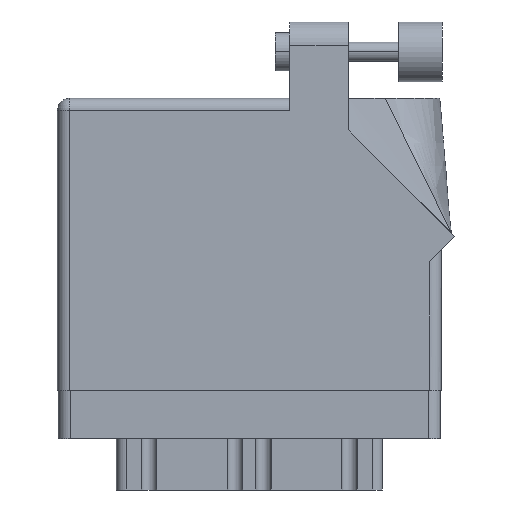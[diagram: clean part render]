
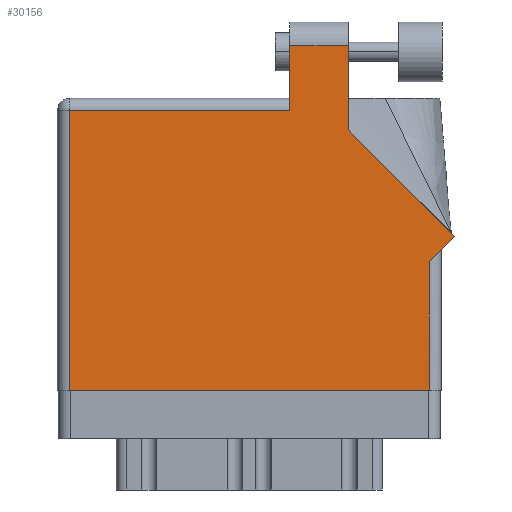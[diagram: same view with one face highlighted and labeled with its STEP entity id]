
A CAD part, front view. The second image highlights one B-rep face of the part: STEP entity #30156.
In plain terms, the highlighted face is planar.
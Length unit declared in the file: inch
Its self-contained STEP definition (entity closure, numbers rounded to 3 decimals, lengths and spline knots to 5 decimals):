
#331 = VECTOR ( 'NONE', #9564, 39.37008 ) ;
#849 = EDGE_CURVE ( 'NONE', #10601, #21095, #9066, .T. ) ;
#1721 = ORIENTED_EDGE ( 'NONE', *, *, #27608, .T. ) ;
#2180 = VECTOR ( 'NONE', #33624, 39.37008 ) ;
#2237 = ORIENTED_EDGE ( 'NONE', *, *, #849, .T. ) ;
#2464 = ORIENTED_EDGE ( 'NONE', *, *, #19576, .T. ) ;
#2592 = EDGE_CURVE ( 'NONE', #9937, #19014, #38317, .T. ) ;
#3768 = VECTOR ( 'NONE', #22594, 39.37008 ) ;
#4319 = CARTESIAN_POINT ( 'NONE',  ( 0.062, 0., 0. ) ) ;
#4365 = LINE ( 'NONE', #37009, #14744 ) ;
#4384 = CARTESIAN_POINT ( 'NONE',  ( 0., 1.53, 0. ) ) ;
#5187 = VERTEX_POINT ( 'NONE', #9441 ) ;
#5222 = ORIENTED_EDGE ( 'NONE', *, *, #8848, .T. ) ;
#5607 = CARTESIAN_POINT ( 'NONE',  ( 1.217, 1.53, 0. ) ) ;
#6119 = CARTESIAN_POINT ( 'NONE',  ( 0., 0., 0. ) ) ;
#6623 = EDGE_CURVE ( 'NONE', #9604, #5187, #30969, .T. ) ;
#6804 = CARTESIAN_POINT ( 'NONE',  ( 1.524, 1.36442, 0. ) ) ;
#7045 = LINE ( 'NONE', #19038, #22514 ) ;
#8455 = LINE ( 'NONE', #38750, #11746 ) ;
#8848 = EDGE_CURVE ( 'NONE', #19730, #20784, #20540, .T. ) ;
#9066 = LINE ( 'NONE', #6119, #2180 ) ;
#9441 = CARTESIAN_POINT ( 'NONE',  ( 1.524, 1.805, 0. ) ) ;
#9564 = DIRECTION ( 'NONE',  ( 0., 1., 0. ) ) ;
#9604 = VERTEX_POINT ( 'NONE', #27274 ) ;
#9704 = FACE_OUTER_BOUND ( 'NONE', #33405, .T. ) ;
#9937 = VERTEX_POINT ( 'NONE', #25664 ) ;
#10103 = CARTESIAN_POINT ( 'NONE',  ( 1.217, 1.468, 0. ) ) ;
#10601 = VERTEX_POINT ( 'NONE', #30463 ) ;
#10674 = VECTOR ( 'NONE', #21131, 39.37008 ) ;
#11167 = DIRECTION ( 'NONE',  ( 0.707, 0.707, 0. ) ) ;
#11746 = VECTOR ( 'NONE', #29871, 39.37008 ) ;
#12852 = DIRECTION ( 'NONE',  ( -1., 0., 0. ) ) ;
#13882 = EDGE_CURVE ( 'NONE', #20784, #26815, #8455, .T. ) ;
#14535 = ORIENTED_EDGE ( 'NONE', *, *, #6623, .T. ) ;
#14567 = DIRECTION ( 'NONE',  ( 0., 1., 0. ) ) ;
#14744 = VECTOR ( 'NONE', #22443, 39.37008 ) ;
#14761 = LINE ( 'NONE', #29287, #33579 ) ;
#15533 = AXIS2_PLACEMENT_3D ( 'NONE', #4384, #16373, #12852 ) ;
#16088 = DIRECTION ( 'NONE',  ( -0.707, 0.707, 0. ) ) ;
#16373 = DIRECTION ( 'NONE',  ( 0., 0., -1. ) ) ;
#19014 = VERTEX_POINT ( 'NONE', #31426 ) ;
#19038 = CARTESIAN_POINT ( 'NONE',  ( 2.08071, 0.80771, 0. ) ) ;
#19576 = EDGE_CURVE ( 'NONE', #26815, #10601, #28661, .T. ) ;
#19730 = VERTEX_POINT ( 'NONE', #38520 ) ;
#20540 = LINE ( 'NONE', #5607, #10674 ) ;
#20784 = VERTEX_POINT ( 'NONE', #10103 ) ;
#20887 = CARTESIAN_POINT ( 'NONE',  ( 1.948, 0., 0. ) ) ;
#21095 = VERTEX_POINT ( 'NONE', #20887 ) ;
#21131 = DIRECTION ( 'NONE',  ( 0., -1., 0. ) ) ;
#21914 = CARTESIAN_POINT ( 'NONE',  ( 0.062, 1.468, 0. ) ) ;
#22443 = DIRECTION ( 'NONE',  ( -1., 0., 0. ) ) ;
#22514 = VECTOR ( 'NONE', #16088, 39.37008 ) ;
#22594 = DIRECTION ( 'NONE',  ( 0., -1., 0. ) ) ;
#25664 = CARTESIAN_POINT ( 'NONE',  ( 1.948, 0.675, 0. ) ) ;
#26815 = VERTEX_POINT ( 'NONE', #21914 ) ;
#27274 = CARTESIAN_POINT ( 'NONE',  ( 1.524, 1.36442, 0. ) ) ;
#27559 = EDGE_CURVE ( 'NONE', #5187, #19730, #4365, .T. ) ;
#27608 = EDGE_CURVE ( 'NONE', #21095, #9937, #14761, .T. ) ;
#28661 = LINE ( 'NONE', #4319, #3768 ) ;
#28802 = ORIENTED_EDGE ( 'NONE', *, *, #13882, .T. ) ;
#29287 = CARTESIAN_POINT ( 'NONE',  ( 1.948, 0.737, 0. ) ) ;
#29362 = ORIENTED_EDGE ( 'NONE', *, *, #2592, .T. ) ;
#29784 = ORIENTED_EDGE ( 'NONE', *, *, #27559, .T. ) ;
#29871 = DIRECTION ( 'NONE',  ( -1., 0., 0. ) ) ;
#30156 = ADVANCED_FACE ( 'NONE', ( #9704 ), #36646, .F. ) ;
#30463 = CARTESIAN_POINT ( 'NONE',  ( 0.062, 0., 0. ) ) ;
#30969 = LINE ( 'NONE', #6804, #331 ) ;
#31062 = EDGE_CURVE ( 'NONE', #19014, #9604, #7045, .T. ) ;
#31426 = CARTESIAN_POINT ( 'NONE',  ( 2.08071, 0.80771, 0. ) ) ;
#33405 = EDGE_LOOP ( 'NONE', ( #14535, #29784, #5222, #28802, #2464, #2237, #1721, #29362, #34738 ) ) ;
#33579 = VECTOR ( 'NONE', #14567, 39.37008 ) ;
#33624 = DIRECTION ( 'NONE',  ( 1., 0., 0. ) ) ;
#34289 = VECTOR ( 'NONE', #11167, 39.37008 ) ;
#34738 = ORIENTED_EDGE ( 'NONE', *, *, #31062, .T. ) ;
#36646 = PLANE ( 'NONE',  #15533 ) ;
#37009 = CARTESIAN_POINT ( 'NONE',  ( 1.217, 1.805, 0. ) ) ;
#38112 = CARTESIAN_POINT ( 'NONE',  ( 2.01, 0.737, 0. ) ) ;
#38317 = LINE ( 'NONE', #38112, #34289 ) ;
#38520 = CARTESIAN_POINT ( 'NONE',  ( 1.217, 1.805, 0. ) ) ;
#38750 = CARTESIAN_POINT ( 'NONE',  ( 0., 1.468, 0. ) ) ;
